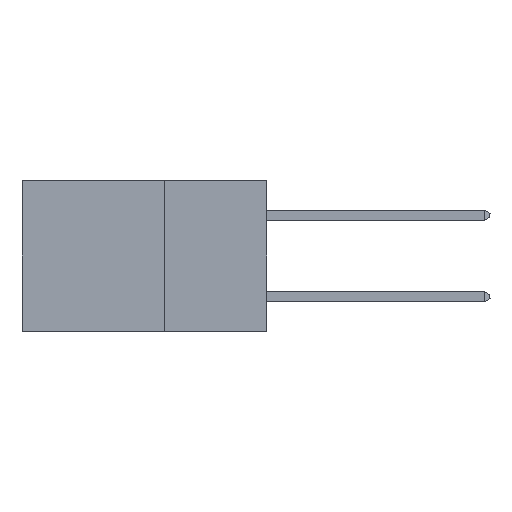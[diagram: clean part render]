
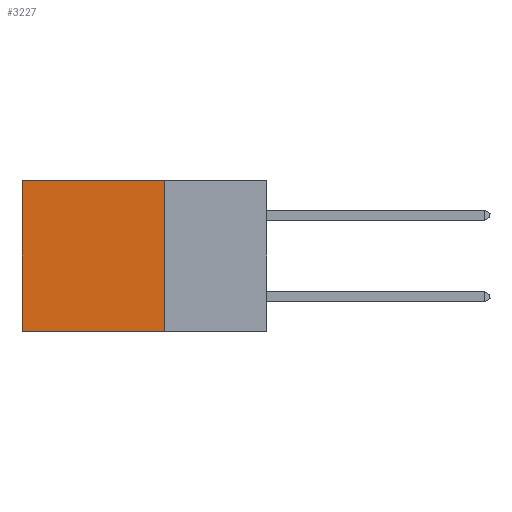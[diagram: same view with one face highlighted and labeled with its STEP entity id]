
A CAD part, left-side view. The second image highlights one B-rep face of the part: STEP entity #3227.
In plain terms, the highlighted planar face has unit normal (-1, 0, 0).
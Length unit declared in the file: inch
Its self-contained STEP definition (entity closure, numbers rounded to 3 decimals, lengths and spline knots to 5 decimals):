
#4 = CARTESIAN_POINT ( 'NONE',  ( 0.2875, 0.6, 0. ) ) ;
#406 = LINE ( 'NONE', #13681, #13478 ) ;
#1467 = DIRECTION ( 'NONE',  ( 1., 0., 0. ) ) ;
#1610 = EDGE_CURVE ( 'NONE', #14941, #15409, #406, .T. ) ;
#1704 = VECTOR ( 'NONE', #15762, 39.37008 ) ;
#2230 = CARTESIAN_POINT ( 'NONE',  ( 0.2875, 0.25, 0. ) ) ;
#3227 = ADVANCED_FACE ( 'NONE', ( #7056 ), #11690, .F. ) ;
#3638 = CARTESIAN_POINT ( 'NONE',  ( 0.2875, 0.6, 0. ) ) ;
#3923 = ORIENTED_EDGE ( 'NONE', *, *, #15533, .F. ) ;
#4768 = EDGE_CURVE ( 'NONE', #15409, #21530, #8280, .T. ) ;
#6058 = VECTOR ( 'NONE', #20517, 39.37008 ) ;
#6293 = LINE ( 'NONE', #2230, #1704 ) ;
#7042 = DIRECTION ( 'NONE',  ( 0., 0., -1. ) ) ;
#7056 = FACE_OUTER_BOUND ( 'NONE', #14051, .T. ) ;
#8029 = ORIENTED_EDGE ( 'NONE', *, *, #1610, .T. ) ;
#8280 = LINE ( 'NONE', #3638, #17727 ) ;
#8696 = CARTESIAN_POINT ( 'NONE',  ( 0.2875, 0.6, -0.37 ) ) ;
#9965 = CARTESIAN_POINT ( 'NONE',  ( 0.2875, 0.25, 0. ) ) ;
#10557 = CARTESIAN_POINT ( 'NONE',  ( 0.2875, 0.25, -0.37 ) ) ;
#10570 = ORIENTED_EDGE ( 'NONE', *, *, #10927, .F. ) ;
#10927 = EDGE_CURVE ( 'NONE', #14941, #14294, #6293, .T. ) ;
#11690 = PLANE ( 'NONE',  #20439 ) ;
#12171 = ORIENTED_EDGE ( 'NONE', *, *, #4768, .T. ) ;
#13392 = DIRECTION ( 'NONE',  ( 0., 0., -1. ) ) ;
#13478 = VECTOR ( 'NONE', #13712, 39.37008 ) ;
#13681 = CARTESIAN_POINT ( 'NONE',  ( 0.2875, 0.25, 0. ) ) ;
#13712 = DIRECTION ( 'NONE',  ( 0., 1., 0. ) ) ;
#14051 = EDGE_LOOP ( 'NONE', ( #12171, #3923, #10570, #8029 ) ) ;
#14294 = VERTEX_POINT ( 'NONE', #19132 ) ;
#14941 = VERTEX_POINT ( 'NONE', #20691 ) ;
#15409 = VERTEX_POINT ( 'NONE', #4 ) ;
#15533 = EDGE_CURVE ( 'NONE', #14294, #21530, #18397, .T. ) ;
#15762 = DIRECTION ( 'NONE',  ( 0., 0., -1. ) ) ;
#17727 = VECTOR ( 'NONE', #7042, 39.37008 ) ;
#18397 = LINE ( 'NONE', #10557, #6058 ) ;
#19132 = CARTESIAN_POINT ( 'NONE',  ( 0.2875, 0.25, -0.37 ) ) ;
#20439 = AXIS2_PLACEMENT_3D ( 'NONE', #9965, #1467, #13392 ) ;
#20517 = DIRECTION ( 'NONE',  ( 0., 1., 0. ) ) ;
#20691 = CARTESIAN_POINT ( 'NONE',  ( 0.2875, 0.25, 0. ) ) ;
#21530 = VERTEX_POINT ( 'NONE', #8696 ) ;
